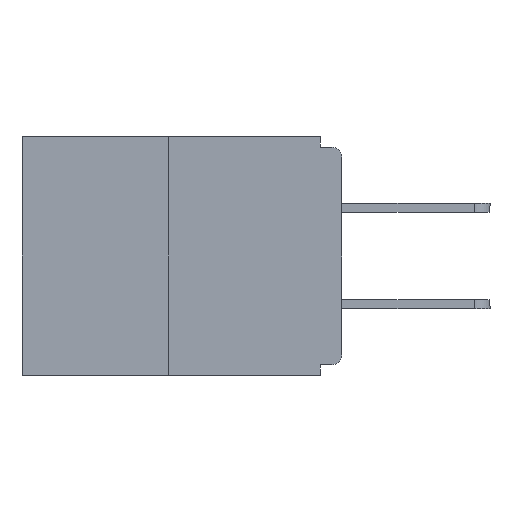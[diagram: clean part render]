
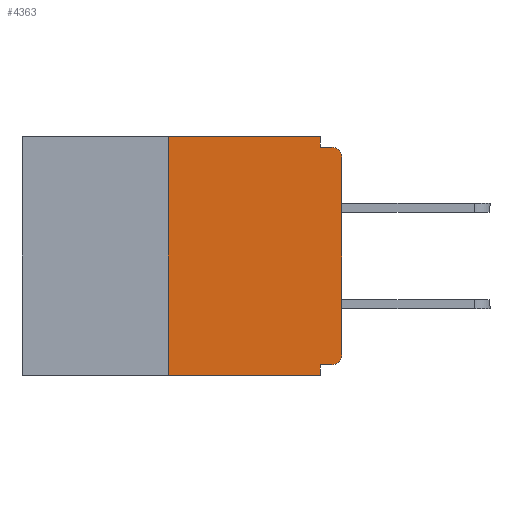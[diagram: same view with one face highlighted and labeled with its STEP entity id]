
A CAD part, left-side view. The second image highlights one B-rep face of the part: STEP entity #4363.
In plain terms, the highlighted planar face has unit normal (-1, 0, 0).
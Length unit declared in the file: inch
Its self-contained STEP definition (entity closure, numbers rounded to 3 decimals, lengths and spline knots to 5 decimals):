
#249 = DIRECTION ( 'NONE',  ( 0., 1., 0. ) ) ;
#259 = CARTESIAN_POINT ( 'NONE',  ( 0., 0.015, -0.313 ) ) ;
#564 = DIRECTION ( 'NONE',  ( 0., 0., -1. ) ) ;
#867 = CIRCLE ( 'NONE', #3914, 0.015 ) ;
#1216 = CARTESIAN_POINT ( 'NONE',  ( 0., 0., -0.03 ) ) ;
#1399 = CARTESIAN_POINT ( 'NONE',  ( 0., 0., -0.015 ) ) ;
#1415 = FACE_OUTER_BOUND ( 'NONE', #16303, .T. ) ;
#1682 = VERTEX_POINT ( 'NONE', #1216 ) ;
#1784 = DIRECTION ( 'NONE',  ( 0., 0., -1. ) ) ;
#1843 = CARTESIAN_POINT ( 'NONE',  ( 0., 0.25, 0. ) ) ;
#2040 = EDGE_CURVE ( 'NONE', #11257, #11355, #10248, .T. ) ;
#2066 = VECTOR ( 'NONE', #14436, 39.37008 ) ;
#2386 = VERTEX_POINT ( 'NONE', #7133 ) ;
#2757 = DIRECTION ( 'NONE',  ( 0., 0., 1. ) ) ;
#3185 = EDGE_CURVE ( 'NONE', #1682, #11434, #10234, .T. ) ;
#3225 = CARTESIAN_POINT ( 'NONE',  ( 0., 0.031, -0.343 ) ) ;
#3462 = EDGE_CURVE ( 'NONE', #11257, #16489, #15660, .T. ) ;
#3754 = ORIENTED_EDGE ( 'NONE', *, *, #10378, .F. ) ;
#3772 = VERTEX_POINT ( 'NONE', #8765 ) ;
#3858 = EDGE_CURVE ( 'NONE', #15247, #11355, #6417, .T. ) ;
#3914 = AXIS2_PLACEMENT_3D ( 'NONE', #259, #6657, #6546 ) ;
#3943 = LINE ( 'NONE', #6574, #15738 ) ;
#3991 = CARTESIAN_POINT ( 'NONE',  ( 0., 0., -0.328 ) ) ;
#4188 = VERTEX_POINT ( 'NONE', #13115 ) ;
#4247 = DIRECTION ( 'NONE',  ( 1., 0., 0. ) ) ;
#4363 = ADVANCED_FACE ( 'NONE', ( #1415 ), #6843, .F. ) ;
#4487 = CARTESIAN_POINT ( 'NONE',  ( 0., 0.031, 0. ) ) ;
#4570 = ORIENTED_EDGE ( 'NONE', *, *, #3462, .F. ) ;
#4769 = CARTESIAN_POINT ( 'NONE',  ( 0., 0.25, 0. ) ) ;
#5244 = DIRECTION ( 'NONE',  ( 0., -1., 0. ) ) ;
#5554 = EDGE_CURVE ( 'NONE', #10995, #4188, #15176, .T. ) ;
#5968 = AXIS2_PLACEMENT_3D ( 'NONE', #10472, #4247, #1784 ) ;
#6212 = ORIENTED_EDGE ( 'NONE', *, *, #3185, .T. ) ;
#6226 = ORIENTED_EDGE ( 'NONE', *, *, #5554, .F. ) ;
#6417 = LINE ( 'NONE', #12255, #11212 ) ;
#6527 = EDGE_CURVE ( 'NONE', #2386, #1682, #3943, .T. ) ;
#6546 = DIRECTION ( 'NONE',  ( 0., 0., -1. ) ) ;
#6574 = CARTESIAN_POINT ( 'NONE',  ( 0., 0., 0. ) ) ;
#6657 = DIRECTION ( 'NONE',  ( -1., 0., 0. ) ) ;
#6817 = ORIENTED_EDGE ( 'NONE', *, *, #16130, .T. ) ;
#6843 = PLANE ( 'NONE',  #5968 ) ;
#7126 = CARTESIAN_POINT ( 'NONE',  ( 0., 0.015, -0.015 ) ) ;
#7133 = CARTESIAN_POINT ( 'NONE',  ( 0., 0., -0.313 ) ) ;
#7421 = CARTESIAN_POINT ( 'NONE',  ( 0., 0.015, -0.03 ) ) ;
#7626 = VECTOR ( 'NONE', #2757, 39.37008 ) ;
#8070 = AXIS2_PLACEMENT_3D ( 'NONE', #7421, #8938, #11515 ) ;
#8298 = LINE ( 'NONE', #1399, #11526 ) ;
#8308 = EDGE_CURVE ( 'NONE', #3772, #15247, #12061, .T. ) ;
#8428 = ORIENTED_EDGE ( 'NONE', *, *, #11169, .F. ) ;
#8653 = VECTOR ( 'NONE', #249, 39.37008 ) ;
#8765 = CARTESIAN_POINT ( 'NONE',  ( 0., 0.015, -0.328 ) ) ;
#8938 = DIRECTION ( 'NONE',  ( -1., 0., 0. ) ) ;
#9577 = VECTOR ( 'NONE', #11949, 39.37008 ) ;
#10234 = CIRCLE ( 'NONE', #8070, 0.015 ) ;
#10248 = LINE ( 'NONE', #13080, #2066 ) ;
#10298 = DIRECTION ( 'NONE',  ( 0., 0., -1. ) ) ;
#10378 = EDGE_CURVE ( 'NONE', #16489, #10995, #13401, .T. ) ;
#10472 = CARTESIAN_POINT ( 'NONE',  ( 0., 0.46, 0. ) ) ;
#10995 = VERTEX_POINT ( 'NONE', #4487 ) ;
#11169 = EDGE_CURVE ( 'NONE', #4188, #11434, #8298, .T. ) ;
#11212 = VECTOR ( 'NONE', #564, 39.37008 ) ;
#11257 = VERTEX_POINT ( 'NONE', #15599 ) ;
#11355 = VERTEX_POINT ( 'NONE', #3225 ) ;
#11420 = CARTESIAN_POINT ( 'NONE',  ( 0., 0.031, 0. ) ) ;
#11434 = VERTEX_POINT ( 'NONE', #7126 ) ;
#11515 = DIRECTION ( 'NONE',  ( 0., 0., -1. ) ) ;
#11526 = VECTOR ( 'NONE', #5244, 39.37008 ) ;
#11749 = VECTOR ( 'NONE', #10298, 39.37008 ) ;
#11865 = ORIENTED_EDGE ( 'NONE', *, *, #3858, .F. ) ;
#11949 = DIRECTION ( 'NONE',  ( 0., -1., 0. ) ) ;
#12061 = LINE ( 'NONE', #3991, #8653 ) ;
#12255 = CARTESIAN_POINT ( 'NONE',  ( 0., 0.031, -0.343 ) ) ;
#12997 = DIRECTION ( 'NONE',  ( 0., 0., 1. ) ) ;
#13026 = ORIENTED_EDGE ( 'NONE', *, *, #2040, .T. ) ;
#13080 = CARTESIAN_POINT ( 'NONE',  ( 0., 0.46, -0.343 ) ) ;
#13115 = CARTESIAN_POINT ( 'NONE',  ( 0., 0.031, -0.015 ) ) ;
#13401 = LINE ( 'NONE', #16291, #9577 ) ;
#14436 = DIRECTION ( 'NONE',  ( 0., -1., 0. ) ) ;
#14784 = ORIENTED_EDGE ( 'NONE', *, *, #6527, .T. ) ;
#15176 = LINE ( 'NONE', #11420, #11749 ) ;
#15247 = VERTEX_POINT ( 'NONE', #16262 ) ;
#15541 = ORIENTED_EDGE ( 'NONE', *, *, #8308, .F. ) ;
#15599 = CARTESIAN_POINT ( 'NONE',  ( 0., 0.25, -0.343 ) ) ;
#15660 = LINE ( 'NONE', #4769, #7626 ) ;
#15738 = VECTOR ( 'NONE', #12997, 39.37008 ) ;
#16130 = EDGE_CURVE ( 'NONE', #3772, #2386, #867, .T. ) ;
#16262 = CARTESIAN_POINT ( 'NONE',  ( 0., 0.031, -0.328 ) ) ;
#16291 = CARTESIAN_POINT ( 'NONE',  ( 0., 0.46, 0. ) ) ;
#16303 = EDGE_LOOP ( 'NONE', ( #3754, #4570, #13026, #11865, #15541, #6817, #14784, #6212, #8428, #6226 ) ) ;
#16489 = VERTEX_POINT ( 'NONE', #1843 ) ;
